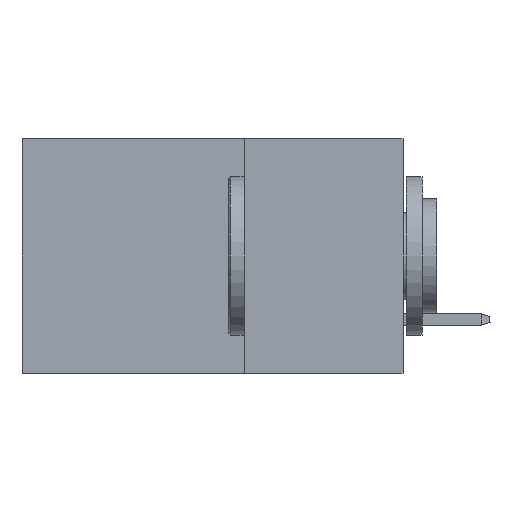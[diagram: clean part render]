
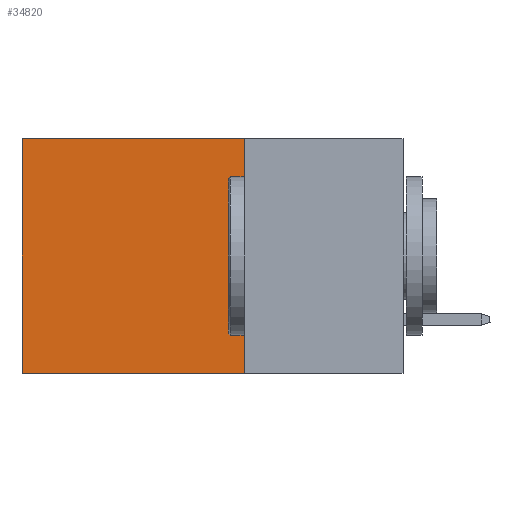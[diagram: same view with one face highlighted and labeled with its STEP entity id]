
A CAD part, left-side view. The second image highlights one B-rep face of the part: STEP entity #34820.
In plain terms, the highlighted planar face has unit normal (-1, 0, 0).
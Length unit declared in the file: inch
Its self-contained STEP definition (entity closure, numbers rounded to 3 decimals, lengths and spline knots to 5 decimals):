
#475 = CARTESIAN_POINT ( 'NONE',  ( 0.2875, 0.25, 0. ) ) ;
#1032 = CARTESIAN_POINT ( 'NONE',  ( 0.2875, 0.25, 0. ) ) ;
#3257 = ORIENTED_EDGE ( 'NONE', *, *, #27209, .T. ) ;
#3717 = VERTEX_POINT ( 'NONE', #24871 ) ;
#5793 = VECTOR ( 'NONE', #20147, 39.37008 ) ;
#6184 = CARTESIAN_POINT ( 'NONE',  ( 0.2875, 0.25, -0.37 ) ) ;
#6962 = CARTESIAN_POINT ( 'NONE',  ( 0.2875, 0.6, 0. ) ) ;
#9515 = VECTOR ( 'NONE', #41611, 39.37008 ) ;
#13414 = VECTOR ( 'NONE', #33349, 39.37008 ) ;
#13674 = EDGE_CURVE ( 'NONE', #25604, #3717, #43881, .T. ) ;
#14286 = ORIENTED_EDGE ( 'NONE', *, *, #32810, .F. ) ;
#14473 = DIRECTION ( 'NONE',  ( 0., 0., -1. ) ) ;
#15767 = DIRECTION ( 'NONE',  ( 1., 0., 0. ) ) ;
#18283 = ORIENTED_EDGE ( 'NONE', *, *, #13674, .T. ) ;
#19576 = CARTESIAN_POINT ( 'NONE',  ( 0.2875, 0.25, 0. ) ) ;
#20147 = DIRECTION ( 'NONE',  ( 0., 1., 0. ) ) ;
#21088 = PLANE ( 'NONE',  #38443 ) ;
#24170 = VERTEX_POINT ( 'NONE', #35243 ) ;
#24364 = LINE ( 'NONE', #6962, #9515 ) ;
#24871 = CARTESIAN_POINT ( 'NONE',  ( 0.2875, 0.6, 0. ) ) ;
#25199 = EDGE_LOOP ( 'NONE', ( #3257, #43185, #14286, #18283 ) ) ;
#25604 = VERTEX_POINT ( 'NONE', #1032 ) ;
#26824 = LINE ( 'NONE', #6184, #5793 ) ;
#27209 = EDGE_CURVE ( 'NONE', #3717, #24170, #24364, .T. ) ;
#29894 = DIRECTION ( 'NONE',  ( 0., 1., 0. ) ) ;
#30113 = CARTESIAN_POINT ( 'NONE',  ( 0.2875, 0.25, 0. ) ) ;
#31459 = VECTOR ( 'NONE', #29894, 39.37008 ) ;
#32427 = VERTEX_POINT ( 'NONE', #44383 ) ;
#32810 = EDGE_CURVE ( 'NONE', #25604, #32427, #41545, .T. ) ;
#33349 = DIRECTION ( 'NONE',  ( 0., 0., -1. ) ) ;
#34820 = ADVANCED_FACE ( 'NONE', ( #35106 ), #21088, .F. ) ;
#35106 = FACE_OUTER_BOUND ( 'NONE', #25199, .T. ) ;
#35243 = CARTESIAN_POINT ( 'NONE',  ( 0.2875, 0.6, -0.37 ) ) ;
#38443 = AXIS2_PLACEMENT_3D ( 'NONE', #475, #15767, #14473 ) ;
#39486 = EDGE_CURVE ( 'NONE', #32427, #24170, #26824, .T. ) ;
#41545 = LINE ( 'NONE', #19576, #13414 ) ;
#41611 = DIRECTION ( 'NONE',  ( 0., 0., -1. ) ) ;
#43185 = ORIENTED_EDGE ( 'NONE', *, *, #39486, .F. ) ;
#43881 = LINE ( 'NONE', #30113, #31459 ) ;
#44383 = CARTESIAN_POINT ( 'NONE',  ( 0.2875, 0.25, -0.37 ) ) ;
